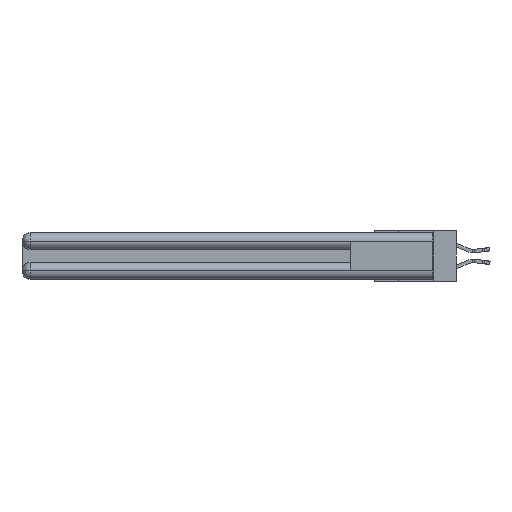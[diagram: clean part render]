
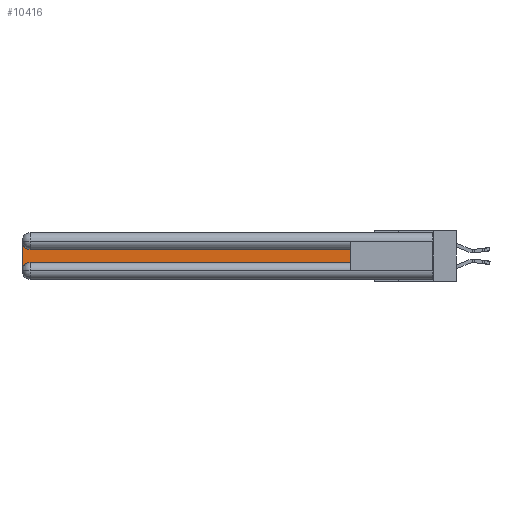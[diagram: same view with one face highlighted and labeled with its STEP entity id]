
A CAD part, left-side view. The second image highlights one B-rep face of the part: STEP entity #10416.
In plain terms, the highlighted planar face has unit normal (-1, 0, 0).
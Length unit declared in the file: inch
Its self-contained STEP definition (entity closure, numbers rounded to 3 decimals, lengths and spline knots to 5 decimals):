
#192 = DIRECTION ( 'NONE',  ( 1., 0., 0. ) ) ;
#432 = AXIS2_PLACEMENT_3D ( 'NONE', #10153, #775, #29292 ) ;
#775 = DIRECTION ( 'NONE',  ( 1., 0., 0. ) ) ;
#1516 = DIRECTION ( 'NONE',  ( 0., 0., -1. ) ) ;
#1649 = CARTESIAN_POINT ( 'NONE',  ( 0.075, 0.6, -0.1225 ) ) ;
#2054 = DIRECTION ( 'NONE',  ( 0., 0., 1. ) ) ;
#2835 = DIRECTION ( 'NONE',  ( 0., 0., -1. ) ) ;
#3111 = EDGE_CURVE ( 'NONE', #10528, #25949, #25294, .T. ) ;
#3750 = CARTESIAN_POINT ( 'NONE',  ( 0.075, 2.94, -0.2175 ) ) ;
#4409 = ORIENTED_EDGE ( 'NONE', *, *, #7418, .T. ) ;
#4834 = CIRCLE ( 'NONE', #432, 0.06 ) ;
#4940 = AXIS2_PLACEMENT_3D ( 'NONE', #21137, #192, #26198 ) ;
#6130 = EDGE_LOOP ( 'NONE', ( #14213, #4409, #26923, #15390, #29591, #28534 ) ) ;
#6626 = PLANE ( 'NONE',  #4940 ) ;
#6648 = DIRECTION ( 'NONE',  ( 0., -1., 0. ) ) ;
#6771 = CIRCLE ( 'NONE', #28564, 0.06 ) ;
#7418 = EDGE_CURVE ( 'NONE', #25341, #19750, #6771, .T. ) ;
#7902 = VERTEX_POINT ( 'NONE', #3750 ) ;
#8182 = CARTESIAN_POINT ( 'NONE',  ( 0.075, 2.94, -0.1225 ) ) ;
#8303 = CARTESIAN_POINT ( 'NONE',  ( 0.075, 0.6, -0.1225 ) ) ;
#8641 = DIRECTION ( 'NONE',  ( 1., 0., 0. ) ) ;
#8934 = CARTESIAN_POINT ( 'NONE',  ( 0.075, 0.6, -0.2175 ) ) ;
#10033 = CARTESIAN_POINT ( 'NONE',  ( 0.075, 3., -0.2175 ) ) ;
#10153 = CARTESIAN_POINT ( 'NONE',  ( 0.075, 2.94, -0.2775 ) ) ;
#10416 = ADVANCED_FACE ( 'NONE', ( #24954 ), #6626, .F. ) ;
#10528 = VERTEX_POINT ( 'NONE', #24744 ) ;
#10626 = VECTOR ( 'NONE', #2835, 39.37008 ) ;
#10931 = CARTESIAN_POINT ( 'NONE',  ( 0.075, 3., -0.0625 ) ) ;
#11347 = CARTESIAN_POINT ( 'NONE',  ( 0.075, 3., -0.2775 ) ) ;
#12075 = EDGE_CURVE ( 'NONE', #22393, #7902, #4834, .T. ) ;
#13939 = LINE ( 'NONE', #10033, #10626 ) ;
#14213 = ORIENTED_EDGE ( 'NONE', *, *, #30459, .T. ) ;
#15390 = ORIENTED_EDGE ( 'NONE', *, *, #12075, .T. ) ;
#18127 = DIRECTION ( 'NONE',  ( 0., 1., 0. ) ) ;
#18624 = VECTOR ( 'NONE', #18127, 39.37008 ) ;
#18642 = EDGE_CURVE ( 'NONE', #19750, #22393, #13939, .T. ) ;
#19058 = VECTOR ( 'NONE', #2054, 39.37008 ) ;
#19750 = VERTEX_POINT ( 'NONE', #10931 ) ;
#21120 = LINE ( 'NONE', #8303, #18624 ) ;
#21137 = CARTESIAN_POINT ( 'NONE',  ( 0.075, 3., -0.1225 ) ) ;
#21458 = CARTESIAN_POINT ( 'NONE',  ( 0.075, 0.6, -0.2175 ) ) ;
#22393 = VERTEX_POINT ( 'NONE', #11347 ) ;
#22848 = LINE ( 'NONE', #8934, #28444 ) ;
#24744 = CARTESIAN_POINT ( 'NONE',  ( 0.075, 0.6, -0.2175 ) ) ;
#24954 = FACE_OUTER_BOUND ( 'NONE', #6130, .T. ) ;
#25252 = CARTESIAN_POINT ( 'NONE',  ( 0.075, 2.94, -0.0625 ) ) ;
#25294 = LINE ( 'NONE', #21458, #19058 ) ;
#25341 = VERTEX_POINT ( 'NONE', #8182 ) ;
#25949 = VERTEX_POINT ( 'NONE', #1649 ) ;
#26198 = DIRECTION ( 'NONE',  ( 0., 0., -1. ) ) ;
#26923 = ORIENTED_EDGE ( 'NONE', *, *, #18642, .T. ) ;
#27097 = EDGE_CURVE ( 'NONE', #7902, #10528, #22848, .T. ) ;
#28444 = VECTOR ( 'NONE', #6648, 39.37008 ) ;
#28534 = ORIENTED_EDGE ( 'NONE', *, *, #3111, .T. ) ;
#28564 = AXIS2_PLACEMENT_3D ( 'NONE', #25252, #8641, #1516 ) ;
#29292 = DIRECTION ( 'NONE',  ( 0., 0., -1. ) ) ;
#29591 = ORIENTED_EDGE ( 'NONE', *, *, #27097, .T. ) ;
#30459 = EDGE_CURVE ( 'NONE', #25949, #25341, #21120, .T. ) ;
